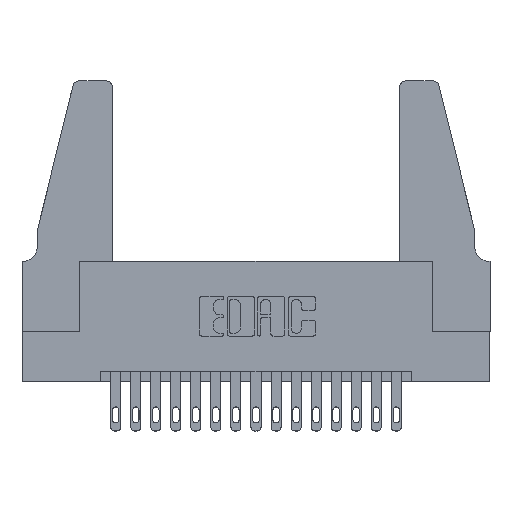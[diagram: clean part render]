
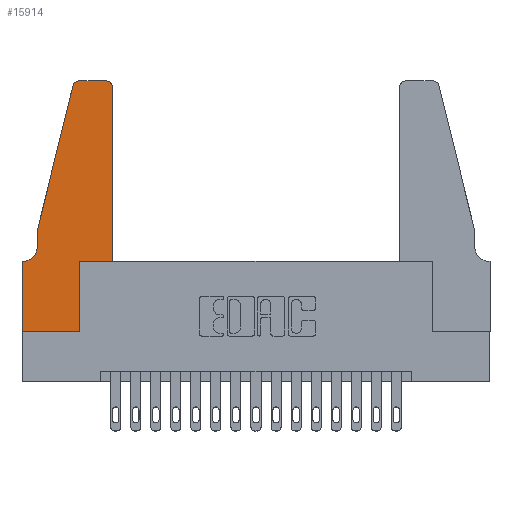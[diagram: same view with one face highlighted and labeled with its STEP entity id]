
A CAD part, top view. The second image highlights one B-rep face of the part: STEP entity #15914.
In plain terms, the highlighted planar face has unit normal (0, 0, 1).
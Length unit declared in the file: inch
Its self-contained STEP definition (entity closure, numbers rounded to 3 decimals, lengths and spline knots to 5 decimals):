
#57 = CARTESIAN_POINT ( 'NONE',  ( 0.4505, 0.35, 0.37 ) ) ;
#233 = VERTEX_POINT ( 'NONE', #7489 ) ;
#296 = VERTEX_POINT ( 'NONE', #17169 ) ;
#427 = DIRECTION ( 'NONE',  ( -1., 0., 0. ) ) ;
#586 = VERTEX_POINT ( 'NONE', #16440 ) ;
#638 = LINE ( 'NONE', #14260, #14585 ) ;
#824 = DIRECTION ( 'NONE',  ( 0., 0., 1. ) ) ;
#877 = DIRECTION ( 'NONE',  ( 0., 1., 0. ) ) ;
#910 = AXIS2_PLACEMENT_3D ( 'NONE', #6816, #6929, #9335 ) ;
#947 = CARTESIAN_POINT ( 'NONE',  ( 0., 0.35, 0.37 ) ) ;
#953 = DIRECTION ( 'NONE',  ( 1., 0., 0. ) ) ;
#1162 = VERTEX_POINT ( 'NONE', #2122 ) ;
#1468 = ORIENTED_EDGE ( 'NONE', *, *, #17313, .T. ) ;
#1555 = FACE_OUTER_BOUND ( 'NONE', #9605, .T. ) ;
#1593 = EDGE_CURVE ( 'NONE', #2647, #586, #16862, .T. ) ;
#1857 = CARTESIAN_POINT ( 'NONE',  ( 0.0755, 0.5, 0.37 ) ) ;
#1912 = ORIENTED_EDGE ( 'NONE', *, *, #9091, .T. ) ;
#2122 = CARTESIAN_POINT ( 'NONE',  ( 0.4505, 0.35, 0.37 ) ) ;
#2296 = VERTEX_POINT ( 'NONE', #4150 ) ;
#2301 = LINE ( 'NONE', #57, #12652 ) ;
#2647 = VERTEX_POINT ( 'NONE', #14329 ) ;
#3111 = CARTESIAN_POINT ( 'NONE',  ( 0.0055, 0.42, 0.37 ) ) ;
#3641 = DIRECTION ( 'NONE',  ( 1., 0., 0. ) ) ;
#3642 = CIRCLE ( 'NONE', #3781, 0.07 ) ;
#3735 = VERTEX_POINT ( 'NONE', #16913 ) ;
#3781 = AXIS2_PLACEMENT_3D ( 'NONE', #3111, #12550, #427 ) ;
#4141 = ORIENTED_EDGE ( 'NONE', *, *, #6371, .T. ) ;
#4150 = CARTESIAN_POINT ( 'NONE',  ( 0.2865, 0., 0.37 ) ) ;
#4204 = CARTESIAN_POINT ( 'NONE',  ( 0.25487, 1.22718, 0.37 ) ) ;
#4208 = VECTOR ( 'NONE', #13134, 39.37008 ) ;
#4547 = CARTESIAN_POINT ( 'NONE',  ( 0.0755, 0.42, 0.37 ) ) ;
#4691 = CARTESIAN_POINT ( 'NONE',  ( 0.4205, 1.22, 0.37 ) ) ;
#5483 = LINE ( 'NONE', #1857, #12027 ) ;
#5527 = LINE ( 'NONE', #15368, #15848 ) ;
#5561 = EDGE_CURVE ( 'NONE', #9148, #8532, #5527, .T. ) ;
#6371 = EDGE_CURVE ( 'NONE', #9895, #14840, #11978, .T. ) ;
#6515 = LINE ( 'NONE', #13806, #9899 ) ;
#6816 = CARTESIAN_POINT ( 'NONE',  ( 0.284, 1.22, 0.37 ) ) ;
#6841 = ORIENTED_EDGE ( 'NONE', *, *, #1593, .T. ) ;
#6929 = DIRECTION ( 'NONE',  ( 0., 0., 1. ) ) ;
#7355 = CARTESIAN_POINT ( 'NONE',  ( 0.0755, 0.35, 0.37 ) ) ;
#7482 = CARTESIAN_POINT ( 'NONE',  ( 0.4505, 0.35, 0.37 ) ) ;
#7489 = CARTESIAN_POINT ( 'NONE',  ( 0.2865, 0.35, 0.37 ) ) ;
#7582 = EDGE_CURVE ( 'NONE', #233, #1162, #7818, .T. ) ;
#7674 = PLANE ( 'NONE',  #11141 ) ;
#7818 = LINE ( 'NONE', #7482, #13541 ) ;
#7819 = EDGE_CURVE ( 'NONE', #296, #2296, #638, .T. ) ;
#7925 = CARTESIAN_POINT ( 'NONE',  ( 0.0755, 0.5, 0.37 ) ) ;
#7960 = LINE ( 'NONE', #10658, #16208 ) ;
#8167 = ORIENTED_EDGE ( 'NONE', *, *, #9732, .T. ) ;
#8532 = VERTEX_POINT ( 'NONE', #7925 ) ;
#8561 = DIRECTION ( 'NONE',  ( 0., -1., 0. ) ) ;
#8711 = EDGE_CURVE ( 'NONE', #8532, #11868, #5483, .T. ) ;
#9026 = DIRECTION ( 'NONE',  ( 0., 0., 1. ) ) ;
#9091 = EDGE_CURVE ( 'NONE', #1162, #2647, #2301, .T. ) ;
#9148 = VERTEX_POINT ( 'NONE', #4204 ) ;
#9281 = ORIENTED_EDGE ( 'NONE', *, *, #7819, .T. ) ;
#9335 = DIRECTION ( 'NONE',  ( 1., 0., 0. ) ) ;
#9406 = DIRECTION ( 'NONE',  ( -1., 0., 0. ) ) ;
#9429 = VECTOR ( 'NONE', #12910, 39.37008 ) ;
#9605 = EDGE_LOOP ( 'NONE', ( #8167, #13968, #10691, #15373, #16767, #4141, #1468, #9281, #14594, #15611, #1912, #6841 ) ) ;
#9707 = DIRECTION ( 'NONE',  ( 0., 1., 0. ) ) ;
#9732 = EDGE_CURVE ( 'NONE', #586, #3735, #7960, .T. ) ;
#9895 = VERTEX_POINT ( 'NONE', #12320 ) ;
#9899 = VECTOR ( 'NONE', #9707, 39.37008 ) ;
#10264 = DIRECTION ( 'NONE',  ( 1., 0., 0. ) ) ;
#10307 = DIRECTION ( 'NONE',  ( 1., 0., 0. ) ) ;
#10604 = CIRCLE ( 'NONE', #910, 0.03 ) ;
#10658 = CARTESIAN_POINT ( 'NONE',  ( 0.2605, 1.25, 0.37 ) ) ;
#10691 = ORIENTED_EDGE ( 'NONE', *, *, #5561, .T. ) ;
#11141 = AXIS2_PLACEMENT_3D ( 'NONE', #17129, #9026, #953 ) ;
#11555 = DIRECTION ( 'NONE',  ( -0.239, -0.971, 0. ) ) ;
#11782 = CARTESIAN_POINT ( 'NONE',  ( 0., 0., 0.37 ) ) ;
#11868 = VERTEX_POINT ( 'NONE', #4547 ) ;
#11978 = LINE ( 'NONE', #7355, #9429 ) ;
#12027 = VECTOR ( 'NONE', #8561, 39.37008 ) ;
#12320 = CARTESIAN_POINT ( 'NONE',  ( 0.0055, 0.35, 0.37 ) ) ;
#12550 = DIRECTION ( 'NONE',  ( 0., 0., -1. ) ) ;
#12552 = AXIS2_PLACEMENT_3D ( 'NONE', #4691, #824, #10264 ) ;
#12652 = VECTOR ( 'NONE', #877, 39.37008 ) ;
#12910 = DIRECTION ( 'NONE',  ( -1., 0., 0. ) ) ;
#13134 = DIRECTION ( 'NONE',  ( 0., -1., 0. ) ) ;
#13541 = VECTOR ( 'NONE', #10307, 39.37008 ) ;
#13806 = CARTESIAN_POINT ( 'NONE',  ( 0.2865, 0.35, 0.37 ) ) ;
#13968 = ORIENTED_EDGE ( 'NONE', *, *, #14284, .T. ) ;
#14260 = CARTESIAN_POINT ( 'NONE',  ( 0., 0., 0.37 ) ) ;
#14284 = EDGE_CURVE ( 'NONE', #3735, #9148, #10604, .T. ) ;
#14329 = CARTESIAN_POINT ( 'NONE',  ( 0.4505, 1.22, 0.37 ) ) ;
#14585 = VECTOR ( 'NONE', #3641, 39.37008 ) ;
#14594 = ORIENTED_EDGE ( 'NONE', *, *, #16821, .T. ) ;
#14840 = VERTEX_POINT ( 'NONE', #947 ) ;
#15368 = CARTESIAN_POINT ( 'NONE',  ( 0.0755, 0.5, 0.37 ) ) ;
#15373 = ORIENTED_EDGE ( 'NONE', *, *, #8711, .T. ) ;
#15611 = ORIENTED_EDGE ( 'NONE', *, *, #7582, .T. ) ;
#15659 = EDGE_CURVE ( 'NONE', #11868, #9895, #3642, .T. ) ;
#15848 = VECTOR ( 'NONE', #11555, 39.37008 ) ;
#15914 = ADVANCED_FACE ( 'NONE', ( #1555 ), #7674, .T. ) ;
#16208 = VECTOR ( 'NONE', #9406, 39.37008 ) ;
#16440 = CARTESIAN_POINT ( 'NONE',  ( 0.4205, 1.25, 0.37 ) ) ;
#16655 = LINE ( 'NONE', #11782, #4208 ) ;
#16767 = ORIENTED_EDGE ( 'NONE', *, *, #15659, .T. ) ;
#16821 = EDGE_CURVE ( 'NONE', #2296, #233, #6515, .T. ) ;
#16862 = CIRCLE ( 'NONE', #12552, 0.03 ) ;
#16913 = CARTESIAN_POINT ( 'NONE',  ( 0.284, 1.25, 0.37 ) ) ;
#17129 = CARTESIAN_POINT ( 'NONE',  ( 0., 0.35, 0.37 ) ) ;
#17169 = CARTESIAN_POINT ( 'NONE',  ( 0., 0., 0.37 ) ) ;
#17313 = EDGE_CURVE ( 'NONE', #14840, #296, #16655, .T. ) ;
